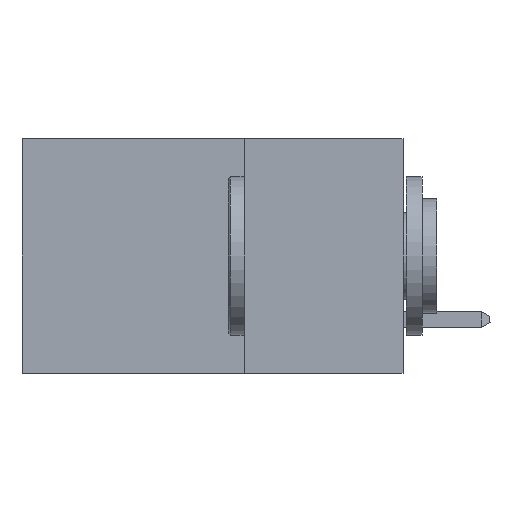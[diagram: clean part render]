
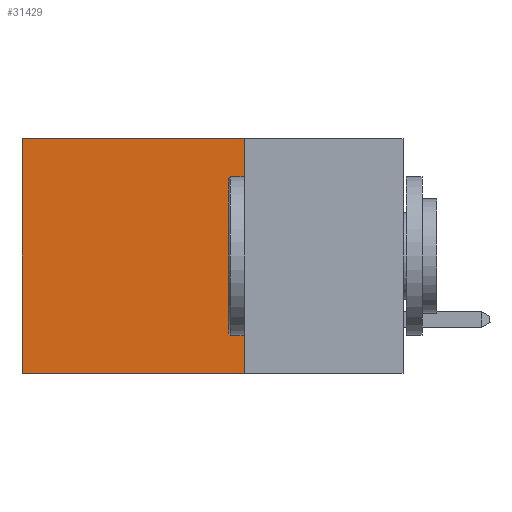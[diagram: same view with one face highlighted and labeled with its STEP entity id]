
A CAD part, left-side view. The second image highlights one B-rep face of the part: STEP entity #31429.
In plain terms, the highlighted planar face has unit normal (-1, 0, 0).
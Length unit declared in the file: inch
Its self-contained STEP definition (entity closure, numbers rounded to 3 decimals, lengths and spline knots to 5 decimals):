
#950 = EDGE_CURVE ( 'NONE', #24169, #6751, #2260, .T. ) ;
#1264 = VECTOR ( 'NONE', #5845, 39.37008 ) ;
#1645 = DIRECTION ( 'NONE',  ( 0., 1., 0. ) ) ;
#2260 = LINE ( 'NONE', #21141, #12102 ) ;
#4896 = LINE ( 'NONE', #7694, #6456 ) ;
#5845 = DIRECTION ( 'NONE',  ( 0., 0., -1. ) ) ;
#6456 = VECTOR ( 'NONE', #37616, 39.37008 ) ;
#6751 = VERTEX_POINT ( 'NONE', #29269 ) ;
#7694 = CARTESIAN_POINT ( 'NONE',  ( 0.2875, 0.25, 0. ) ) ;
#8122 = LINE ( 'NONE', #38551, #28831 ) ;
#8290 = FACE_OUTER_BOUND ( 'NONE', #40696, .T. ) ;
#8544 = LINE ( 'NONE', #12903, #1264 ) ;
#9805 = VERTEX_POINT ( 'NONE', #25949 ) ;
#12102 = VECTOR ( 'NONE', #13883, 39.37008 ) ;
#12903 = CARTESIAN_POINT ( 'NONE',  ( 0.2875, 0.6, 0. ) ) ;
#13883 = DIRECTION ( 'NONE',  ( 0., 0., -1. ) ) ;
#14300 = DIRECTION ( 'NONE',  ( 0., 0., -1. ) ) ;
#14472 = ORIENTED_EDGE ( 'NONE', *, *, #40190, .T. ) ;
#19269 = CARTESIAN_POINT ( 'NONE',  ( 0.2875, 0.6, 0. ) ) ;
#19997 = ORIENTED_EDGE ( 'NONE', *, *, #33073, .F. ) ;
#21141 = CARTESIAN_POINT ( 'NONE',  ( 0.2875, 0.25, 0. ) ) ;
#24169 = VERTEX_POINT ( 'NONE', #29940 ) ;
#24766 = ORIENTED_EDGE ( 'NONE', *, *, #34662, .T. ) ;
#25949 = CARTESIAN_POINT ( 'NONE',  ( 0.2875, 0.6, -0.37 ) ) ;
#26252 = VERTEX_POINT ( 'NONE', #19269 ) ;
#28831 = VECTOR ( 'NONE', #1645, 39.37008 ) ;
#29269 = CARTESIAN_POINT ( 'NONE',  ( 0.2875, 0.25, -0.37 ) ) ;
#29607 = AXIS2_PLACEMENT_3D ( 'NONE', #36900, #30398, #14300 ) ;
#29940 = CARTESIAN_POINT ( 'NONE',  ( 0.2875, 0.25, 0. ) ) ;
#30398 = DIRECTION ( 'NONE',  ( 1., 0., 0. ) ) ;
#31429 = ADVANCED_FACE ( 'NONE', ( #8290 ), #34012, .F. ) ;
#31844 = ORIENTED_EDGE ( 'NONE', *, *, #950, .F. ) ;
#33073 = EDGE_CURVE ( 'NONE', #6751, #9805, #8122, .T. ) ;
#34012 = PLANE ( 'NONE',  #29607 ) ;
#34662 = EDGE_CURVE ( 'NONE', #24169, #26252, #4896, .T. ) ;
#36900 = CARTESIAN_POINT ( 'NONE',  ( 0.2875, 0.25, 0. ) ) ;
#37616 = DIRECTION ( 'NONE',  ( 0., 1., 0. ) ) ;
#38551 = CARTESIAN_POINT ( 'NONE',  ( 0.2875, 0.25, -0.37 ) ) ;
#40190 = EDGE_CURVE ( 'NONE', #26252, #9805, #8544, .T. ) ;
#40696 = EDGE_LOOP ( 'NONE', ( #14472, #19997, #31844, #24766 ) ) ;
